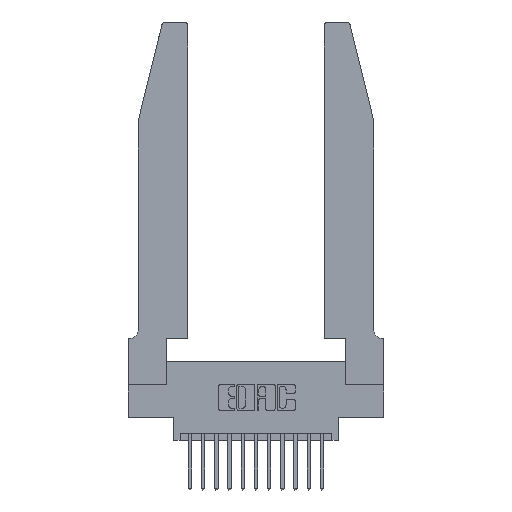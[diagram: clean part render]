
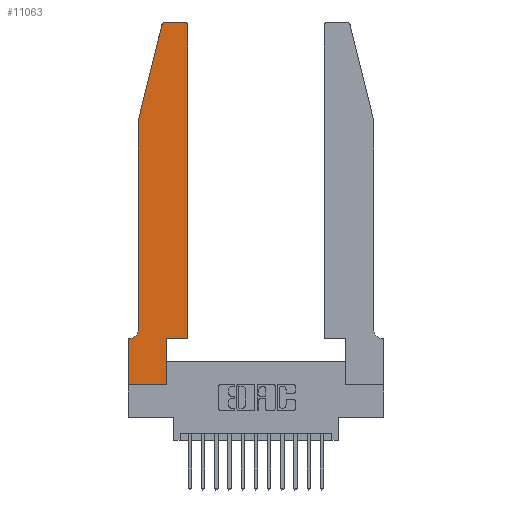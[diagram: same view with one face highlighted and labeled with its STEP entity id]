
A CAD part, top view. The second image highlights one B-rep face of the part: STEP entity #11063.
In plain terms, the highlighted planar face has unit normal (0, 0, 1).
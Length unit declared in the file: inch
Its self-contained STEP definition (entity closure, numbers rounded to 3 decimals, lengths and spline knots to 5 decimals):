
#9 = CARTESIAN_POINT ( 'NONE',  ( 0.0755, 2., 0.37 ) ) ;
#62 = ORIENTED_EDGE ( 'NONE', *, *, #1714, .T. ) ;
#244 = VECTOR ( 'NONE', #17620, 39.37008 ) ;
#549 = DIRECTION ( 'NONE',  ( -0.239, -0.971, 0. ) ) ;
#561 = LINE ( 'NONE', #1733, #4772 ) ;
#564 = ORIENTED_EDGE ( 'NONE', *, *, #5631, .T. ) ;
#586 = CARTESIAN_POINT ( 'NONE',  ( 0.0055, 0.35, 0.37 ) ) ;
#810 = VECTOR ( 'NONE', #8787, 39.37008 ) ;
#930 = VERTEX_POINT ( 'NONE', #2758 ) ;
#1029 = VERTEX_POINT ( 'NONE', #2797 ) ;
#1159 = CARTESIAN_POINT ( 'NONE',  ( 0., 0., 0.37 ) ) ;
#1700 = ORIENTED_EDGE ( 'NONE', *, *, #11448, .T. ) ;
#1714 = EDGE_CURVE ( 'NONE', #17470, #3650, #7886, .T. ) ;
#1733 = CARTESIAN_POINT ( 'NONE',  ( 0.0755, 2., 0.37 ) ) ;
#2277 = CARTESIAN_POINT ( 'NONE',  ( 0.4205, 2.75, 0.37 ) ) ;
#2293 = CARTESIAN_POINT ( 'NONE',  ( 0., 0.35, 0.37 ) ) ;
#2691 = EDGE_CURVE ( 'NONE', #10294, #8620, #12676, .T. ) ;
#2701 = EDGE_CURVE ( 'NONE', #13577, #17551, #11820, .T. ) ;
#2758 = CARTESIAN_POINT ( 'NONE',  ( 0.2865, 0., 0.37 ) ) ;
#2797 = CARTESIAN_POINT ( 'NONE',  ( 0.0755, 0.42, 0.37 ) ) ;
#2957 = EDGE_CURVE ( 'NONE', #3650, #1029, #561, .T. ) ;
#3161 = DIRECTION ( 'NONE',  ( 1., 0., 0. ) ) ;
#3257 = CARTESIAN_POINT ( 'NONE',  ( 0.0755, 2., 0.37 ) ) ;
#3399 = CARTESIAN_POINT ( 'NONE',  ( 0.0055, 0.42, 0.37 ) ) ;
#3650 = VERTEX_POINT ( 'NONE', #3257 ) ;
#4108 = DIRECTION ( 'NONE',  ( 0., 0., 1. ) ) ;
#4337 = ORIENTED_EDGE ( 'NONE', *, *, #13171, .T. ) ;
#4623 = EDGE_CURVE ( 'NONE', #6574, #930, #7623, .T. ) ;
#4772 = VECTOR ( 'NONE', #8902, 39.37008 ) ;
#4798 = DIRECTION ( 'NONE',  ( -1., 0., 0. ) ) ;
#4815 = FACE_OUTER_BOUND ( 'NONE', #16304, .T. ) ;
#5141 = DIRECTION ( 'NONE',  ( 0., 0., 1. ) ) ;
#5287 = CARTESIAN_POINT ( 'NONE',  ( 0.2605, 2.75, 0.37 ) ) ;
#5385 = ORIENTED_EDGE ( 'NONE', *, *, #4623, .T. ) ;
#5594 = LINE ( 'NONE', #8918, #14744 ) ;
#5631 = EDGE_CURVE ( 'NONE', #17551, #13188, #16696, .T. ) ;
#6063 = AXIS2_PLACEMENT_3D ( 'NONE', #6807, #17028, #3161 ) ;
#6101 = CARTESIAN_POINT ( 'NONE',  ( 0.4505, 0.35, 0.37 ) ) ;
#6157 = AXIS2_PLACEMENT_3D ( 'NONE', #3399, #12962, #4798 ) ;
#6235 = ORIENTED_EDGE ( 'NONE', *, *, #16008, .T. ) ;
#6263 = DIRECTION ( 'NONE',  ( 0., 1., 0. ) ) ;
#6357 = VECTOR ( 'NONE', #12119, 39.37008 ) ;
#6452 = CIRCLE ( 'NONE', #13803, 0.03 ) ;
#6574 = VERTEX_POINT ( 'NONE', #15403 ) ;
#6807 = CARTESIAN_POINT ( 'NONE',  ( 0.4205, 2.72, 0.37 ) ) ;
#6847 = CIRCLE ( 'NONE', #6157, 0.07 ) ;
#7252 = VECTOR ( 'NONE', #15126, 39.37008 ) ;
#7478 = ORIENTED_EDGE ( 'NONE', *, *, #2957, .T. ) ;
#7534 = VERTEX_POINT ( 'NONE', #13699 ) ;
#7587 = CARTESIAN_POINT ( 'NONE',  ( 0.4505, 0.35, 0.37 ) ) ;
#7623 = LINE ( 'NONE', #10974, #244 ) ;
#7635 = DIRECTION ( 'NONE',  ( -1., 0., 0. ) ) ;
#7673 = LINE ( 'NONE', #11057, #7252 ) ;
#7886 = LINE ( 'NONE', #9, #14759 ) ;
#8422 = AXIS2_PLACEMENT_3D ( 'NONE', #2293, #5141, #14659 ) ;
#8620 = VERTEX_POINT ( 'NONE', #10711 ) ;
#8787 = DIRECTION ( 'NONE',  ( 1., 0., 0. ) ) ;
#8902 = DIRECTION ( 'NONE',  ( 0., -1., 0. ) ) ;
#8918 = CARTESIAN_POINT ( 'NONE',  ( 0.0755, 0.35, 0.37 ) ) ;
#9371 = ORIENTED_EDGE ( 'NONE', *, *, #15021, .T. ) ;
#10233 = ORIENTED_EDGE ( 'NONE', *, *, #14730, .T. ) ;
#10294 = VERTEX_POINT ( 'NONE', #14567 ) ;
#10711 = CARTESIAN_POINT ( 'NONE',  ( 0.4505, 0.35, 0.37 ) ) ;
#10765 = DIRECTION ( 'NONE',  ( 0., -1., 0. ) ) ;
#10974 = CARTESIAN_POINT ( 'NONE',  ( 0., 0., 0.37 ) ) ;
#11057 = CARTESIAN_POINT ( 'NONE',  ( 0.2865, 0.35, 0.37 ) ) ;
#11063 = ADVANCED_FACE ( 'NONE', ( #4815 ), #13333, .T. ) ;
#11448 = EDGE_CURVE ( 'NONE', #8620, #13577, #13750, .T. ) ;
#11820 = CIRCLE ( 'NONE', #6063, 0.03 ) ;
#12119 = DIRECTION ( 'NONE',  ( -1., 0., 0. ) ) ;
#12310 = CARTESIAN_POINT ( 'NONE',  ( 0.284, 2.72, 0.37 ) ) ;
#12676 = LINE ( 'NONE', #6101, #810 ) ;
#12962 = DIRECTION ( 'NONE',  ( 0., 0., -1. ) ) ;
#13171 = EDGE_CURVE ( 'NONE', #13188, #17470, #6452, .T. ) ;
#13188 = VERTEX_POINT ( 'NONE', #17600 ) ;
#13333 = PLANE ( 'NONE',  #8422 ) ;
#13577 = VERTEX_POINT ( 'NONE', #15718 ) ;
#13652 = DIRECTION ( 'NONE',  ( 1., 0., 0. ) ) ;
#13699 = CARTESIAN_POINT ( 'NONE',  ( 0., 0.35, 0.37 ) ) ;
#13750 = LINE ( 'NONE', #7587, #16821 ) ;
#13803 = AXIS2_PLACEMENT_3D ( 'NONE', #12310, #4108, #13652 ) ;
#14329 = VECTOR ( 'NONE', #10765, 39.37008 ) ;
#14567 = CARTESIAN_POINT ( 'NONE',  ( 0.2865, 0.35, 0.37 ) ) ;
#14659 = DIRECTION ( 'NONE',  ( 1., 0., 0. ) ) ;
#14672 = VERTEX_POINT ( 'NONE', #586 ) ;
#14730 = EDGE_CURVE ( 'NONE', #14672, #7534, #5594, .T. ) ;
#14744 = VECTOR ( 'NONE', #7635, 39.37008 ) ;
#14759 = VECTOR ( 'NONE', #549, 39.37008 ) ;
#15021 = EDGE_CURVE ( 'NONE', #930, #10294, #7673, .T. ) ;
#15126 = DIRECTION ( 'NONE',  ( 0., 1., 0. ) ) ;
#15360 = ORIENTED_EDGE ( 'NONE', *, *, #2701, .T. ) ;
#15403 = CARTESIAN_POINT ( 'NONE',  ( 0., 0., 0.37 ) ) ;
#15718 = CARTESIAN_POINT ( 'NONE',  ( 0.4505, 2.72, 0.37 ) ) ;
#15769 = ORIENTED_EDGE ( 'NONE', *, *, #2691, .T. ) ;
#15818 = EDGE_CURVE ( 'NONE', #1029, #14672, #6847, .T. ) ;
#16008 = EDGE_CURVE ( 'NONE', #7534, #6574, #17371, .T. ) ;
#16304 = EDGE_LOOP ( 'NONE', ( #564, #4337, #62, #7478, #16999, #10233, #6235, #5385, #9371, #15769, #1700, #15360 ) ) ;
#16696 = LINE ( 'NONE', #5287, #6357 ) ;
#16821 = VECTOR ( 'NONE', #6263, 39.37008 ) ;
#16999 = ORIENTED_EDGE ( 'NONE', *, *, #15818, .T. ) ;
#17028 = DIRECTION ( 'NONE',  ( 0., 0., 1. ) ) ;
#17046 = CARTESIAN_POINT ( 'NONE',  ( 0.25487, 2.72718, 0.37 ) ) ;
#17371 = LINE ( 'NONE', #1159, #14329 ) ;
#17470 = VERTEX_POINT ( 'NONE', #17046 ) ;
#17551 = VERTEX_POINT ( 'NONE', #2277 ) ;
#17600 = CARTESIAN_POINT ( 'NONE',  ( 0.284, 2.75, 0.37 ) ) ;
#17620 = DIRECTION ( 'NONE',  ( 1., 0., 0. ) ) ;
